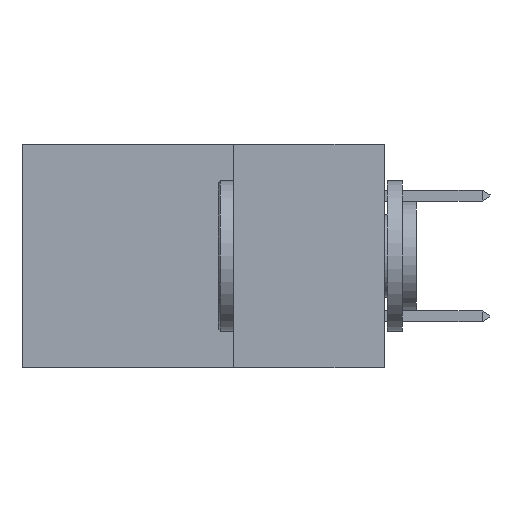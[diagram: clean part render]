
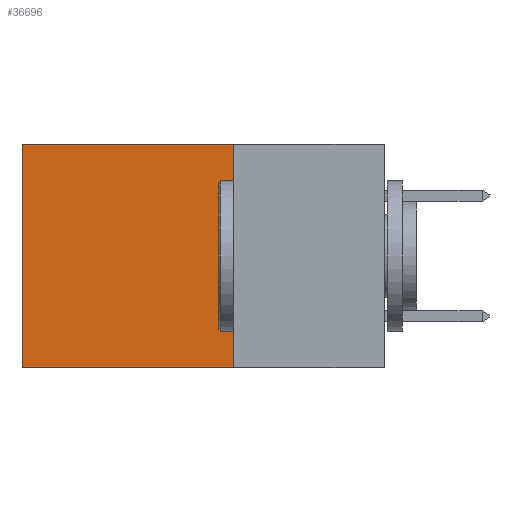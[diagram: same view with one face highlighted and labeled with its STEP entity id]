
A CAD part, left-side view. The second image highlights one B-rep face of the part: STEP entity #36696.
In plain terms, the highlighted planar face has unit normal (-1, 0, 0).
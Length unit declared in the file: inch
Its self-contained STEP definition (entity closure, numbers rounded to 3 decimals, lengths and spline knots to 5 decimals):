
#2086 = CARTESIAN_POINT ( 'NONE',  ( 0.2875, 0.6, 0. ) ) ;
#2259 = ORIENTED_EDGE ( 'NONE', *, *, #34131, .F. ) ;
#3293 = FACE_OUTER_BOUND ( 'NONE', #24023, .T. ) ;
#3879 = EDGE_CURVE ( 'NONE', #32607, #36994, #34304, .T. ) ;
#4189 = VECTOR ( 'NONE', #28916, 39.37008 ) ;
#5380 = LINE ( 'NONE', #14293, #12493 ) ;
#6148 = EDGE_CURVE ( 'NONE', #30043, #12565, #10738, .T. ) ;
#6164 = ORIENTED_EDGE ( 'NONE', *, *, #6148, .T. ) ;
#7922 = CARTESIAN_POINT ( 'NONE',  ( 0.2875, 0.25, 0. ) ) ;
#10738 = LINE ( 'NONE', #2086, #17757 ) ;
#12493 = VECTOR ( 'NONE', #17331, 39.37008 ) ;
#12565 = VERTEX_POINT ( 'NONE', #13653 ) ;
#12853 = CARTESIAN_POINT ( 'NONE',  ( 0.2875, 0.25, 0. ) ) ;
#13415 = LINE ( 'NONE', #36710, #28384 ) ;
#13653 = CARTESIAN_POINT ( 'NONE',  ( 0.2875, 0.6, -0.37 ) ) ;
#14293 = CARTESIAN_POINT ( 'NONE',  ( 0.2875, 0.25, 0. ) ) ;
#15176 = ORIENTED_EDGE ( 'NONE', *, *, #38528, .T. ) ;
#15863 = DIRECTION ( 'NONE',  ( 0., 0., -1. ) ) ;
#17331 = DIRECTION ( 'NONE',  ( 0., 1., 0. ) ) ;
#17757 = VECTOR ( 'NONE', #26081, 39.37008 ) ;
#18258 = ORIENTED_EDGE ( 'NONE', *, *, #3879, .F. ) ;
#19503 = AXIS2_PLACEMENT_3D ( 'NONE', #12853, #33807, #15863 ) ;
#21778 = PLANE ( 'NONE',  #19503 ) ;
#21800 = DIRECTION ( 'NONE',  ( 0., 1., 0. ) ) ;
#23311 = CARTESIAN_POINT ( 'NONE',  ( 0.2875, 0.25, -0.37 ) ) ;
#24023 = EDGE_LOOP ( 'NONE', ( #6164, #2259, #18258, #15176 ) ) ;
#26081 = DIRECTION ( 'NONE',  ( 0., 0., -1. ) ) ;
#28384 = VECTOR ( 'NONE', #21800, 39.37008 ) ;
#28916 = DIRECTION ( 'NONE',  ( 0., 0., -1. ) ) ;
#30043 = VERTEX_POINT ( 'NONE', #38049 ) ;
#32607 = VERTEX_POINT ( 'NONE', #35889 ) ;
#33807 = DIRECTION ( 'NONE',  ( 1., 0., 0. ) ) ;
#34131 = EDGE_CURVE ( 'NONE', #36994, #12565, #13415, .T. ) ;
#34304 = LINE ( 'NONE', #7922, #4189 ) ;
#35889 = CARTESIAN_POINT ( 'NONE',  ( 0.2875, 0.25, 0. ) ) ;
#36696 = ADVANCED_FACE ( 'NONE', ( #3293 ), #21778, .F. ) ;
#36710 = CARTESIAN_POINT ( 'NONE',  ( 0.2875, 0.25, -0.37 ) ) ;
#36994 = VERTEX_POINT ( 'NONE', #23311 ) ;
#38049 = CARTESIAN_POINT ( 'NONE',  ( 0.2875, 0.6, 0. ) ) ;
#38528 = EDGE_CURVE ( 'NONE', #32607, #30043, #5380, .T. ) ;
